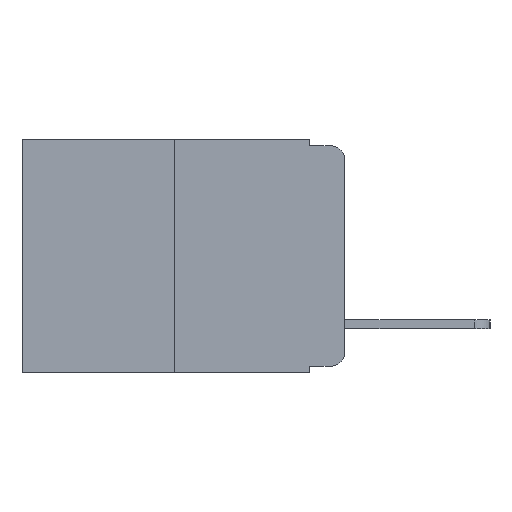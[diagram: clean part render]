
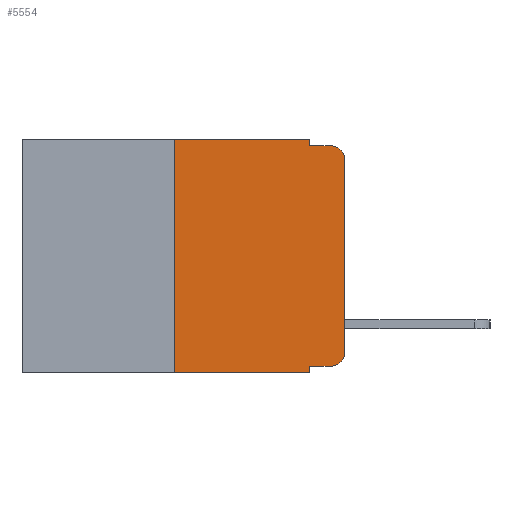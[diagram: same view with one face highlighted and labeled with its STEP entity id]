
A CAD part, left-side view. The second image highlights one B-rep face of the part: STEP entity #5554.
In plain terms, the highlighted planar face has unit normal (-1, 0, 0).
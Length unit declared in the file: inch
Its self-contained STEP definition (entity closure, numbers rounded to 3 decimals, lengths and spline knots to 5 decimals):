
#55 = EDGE_LOOP ( 'NONE', ( #23226, #8332, #12631, #1356, #17486, #22641, #6221, #17511, #11118, #7426 ) ) ;
#192 = VECTOR ( 'NONE', #3516, 39.37008 ) ;
#468 = CARTESIAN_POINT ( 'NONE',  ( 0., 0.02, -0.333 ) ) ;
#478 = VECTOR ( 'NONE', #23734, 39.37008 ) ;
#829 = EDGE_CURVE ( 'NONE', #23364, #8058, #15753, .T. ) ;
#837 = DIRECTION ( 'NONE',  ( -1., 0., 0. ) ) ;
#1308 = DIRECTION ( 'NONE',  ( -1., 0., 0. ) ) ;
#1338 = DIRECTION ( 'NONE',  ( 0., 0., -1. ) ) ;
#1356 = ORIENTED_EDGE ( 'NONE', *, *, #12495, .F. ) ;
#1454 = CARTESIAN_POINT ( 'NONE',  ( 0., 0.02, -0.03 ) ) ;
#2047 = CIRCLE ( 'NONE', #23955, 0.02 ) ;
#2201 = CARTESIAN_POINT ( 'NONE',  ( 0., 0.051, -0.333 ) ) ;
#3516 = DIRECTION ( 'NONE',  ( 0., 0., 1. ) ) ;
#3581 = CARTESIAN_POINT ( 'NONE',  ( 0., 0.473, 0. ) ) ;
#3917 = AXIS2_PLACEMENT_3D ( 'NONE', #19234, #21228, #9553 ) ;
#4253 = EDGE_CURVE ( 'NONE', #8058, #16435, #22614, .T. ) ;
#4354 = CARTESIAN_POINT ( 'NONE',  ( 0., 0.051, -0.343 ) ) ;
#4356 = LINE ( 'NONE', #15771, #24392 ) ;
#5285 = VECTOR ( 'NONE', #11398, 39.37008 ) ;
#5506 = DIRECTION ( 'NONE',  ( 0., -1., 0. ) ) ;
#5554 = ADVANCED_FACE ( 'NONE', ( #6406 ), #13431, .F. ) ;
#5944 = EDGE_CURVE ( 'NONE', #13067, #16435, #12203, .T. ) ;
#6221 = ORIENTED_EDGE ( 'NONE', *, *, #21981, .T. ) ;
#6253 = CARTESIAN_POINT ( 'NONE',  ( 0., 0., 0. ) ) ;
#6406 = FACE_OUTER_BOUND ( 'NONE', #55, .T. ) ;
#6565 = VERTEX_POINT ( 'NONE', #14674 ) ;
#6851 = LINE ( 'NONE', #21825, #478 ) ;
#7160 = CARTESIAN_POINT ( 'NONE',  ( 0., 0., -0.313 ) ) ;
#7342 = DIRECTION ( 'NONE',  ( 0., 0., -1. ) ) ;
#7426 = ORIENTED_EDGE ( 'NONE', *, *, #19051, .T. ) ;
#7667 = LINE ( 'NONE', #11842, #17429 ) ;
#8058 = VERTEX_POINT ( 'NONE', #21269 ) ;
#8332 = ORIENTED_EDGE ( 'NONE', *, *, #4253, .T. ) ;
#8640 = EDGE_CURVE ( 'NONE', #11841, #11509, #6851, .T. ) ;
#8820 = VECTOR ( 'NONE', #7342, 39.37008 ) ;
#9287 = LINE ( 'NONE', #25022, #24155 ) ;
#9553 = DIRECTION ( 'NONE',  ( 0., 0., -1. ) ) ;
#11118 = ORIENTED_EDGE ( 'NONE', *, *, #20085, .T. ) ;
#11398 = DIRECTION ( 'NONE',  ( 0., -1., 0. ) ) ;
#11509 = VERTEX_POINT ( 'NONE', #24253 ) ;
#11786 = CARTESIAN_POINT ( 'NONE',  ( 0., 0.25, -0.343 ) ) ;
#11840 = DIRECTION ( 'NONE',  ( 0., -1., 0. ) ) ;
#11841 = VERTEX_POINT ( 'NONE', #11786 ) ;
#11842 = CARTESIAN_POINT ( 'NONE',  ( 0., 0.051, 0. ) ) ;
#11906 = CARTESIAN_POINT ( 'NONE',  ( 0., 0.051, -0.01 ) ) ;
#12203 = LINE ( 'NONE', #24288, #17358 ) ;
#12495 = EDGE_CURVE ( 'NONE', #6565, #13067, #7667, .T. ) ;
#12499 = CARTESIAN_POINT ( 'NONE',  ( 0., 0.02, -0.313 ) ) ;
#12631 = ORIENTED_EDGE ( 'NONE', *, *, #5944, .F. ) ;
#13067 = VERTEX_POINT ( 'NONE', #11906 ) ;
#13287 = CARTESIAN_POINT ( 'NONE',  ( 0., 0.051, 0. ) ) ;
#13431 = PLANE ( 'NONE',  #3917 ) ;
#13839 = DIRECTION ( 'NONE',  ( 0., 0., -1. ) ) ;
#14497 = DIRECTION ( 'NONE',  ( 0., 0., -1. ) ) ;
#14672 = LINE ( 'NONE', #13287, #8820 ) ;
#14674 = CARTESIAN_POINT ( 'NONE',  ( 0., 0.051, 0. ) ) ;
#14913 = VERTEX_POINT ( 'NONE', #2201 ) ;
#15098 = LINE ( 'NONE', #3581, #5285 ) ;
#15753 = LINE ( 'NONE', #6253, #192 ) ;
#15771 = CARTESIAN_POINT ( 'NONE',  ( 0., 0.473, -0.343 ) ) ;
#16435 = VERTEX_POINT ( 'NONE', #20655 ) ;
#17358 = VECTOR ( 'NONE', #18468, 39.37008 ) ;
#17429 = VECTOR ( 'NONE', #13839, 39.37008 ) ;
#17476 = EDGE_CURVE ( 'NONE', #14913, #23680, #14672, .T. ) ;
#17486 = ORIENTED_EDGE ( 'NONE', *, *, #20573, .F. ) ;
#17511 = ORIENTED_EDGE ( 'NONE', *, *, #17476, .F. ) ;
#17702 = VERTEX_POINT ( 'NONE', #468 ) ;
#18468 = DIRECTION ( 'NONE',  ( 0., -1., 0. ) ) ;
#19051 = EDGE_CURVE ( 'NONE', #17702, #23364, #2047, .T. ) ;
#19234 = CARTESIAN_POINT ( 'NONE',  ( 0., 0.473, 0. ) ) ;
#20085 = EDGE_CURVE ( 'NONE', #14913, #17702, #9287, .T. ) ;
#20573 = EDGE_CURVE ( 'NONE', #11509, #6565, #15098, .T. ) ;
#20655 = CARTESIAN_POINT ( 'NONE',  ( 0., 0.02, -0.01 ) ) ;
#20695 = AXIS2_PLACEMENT_3D ( 'NONE', #1454, #1308, #1338 ) ;
#21228 = DIRECTION ( 'NONE',  ( 1., 0., 0. ) ) ;
#21269 = CARTESIAN_POINT ( 'NONE',  ( 0., 0., -0.03 ) ) ;
#21825 = CARTESIAN_POINT ( 'NONE',  ( 0., 0.25, 0. ) ) ;
#21981 = EDGE_CURVE ( 'NONE', #11841, #23680, #4356, .T. ) ;
#22614 = CIRCLE ( 'NONE', #20695, 0.02 ) ;
#22641 = ORIENTED_EDGE ( 'NONE', *, *, #8640, .F. ) ;
#23226 = ORIENTED_EDGE ( 'NONE', *, *, #829, .T. ) ;
#23364 = VERTEX_POINT ( 'NONE', #7160 ) ;
#23680 = VERTEX_POINT ( 'NONE', #4354 ) ;
#23734 = DIRECTION ( 'NONE',  ( 0., 0., 1. ) ) ;
#23955 = AXIS2_PLACEMENT_3D ( 'NONE', #12499, #837, #14497 ) ;
#24155 = VECTOR ( 'NONE', #5506, 39.37008 ) ;
#24253 = CARTESIAN_POINT ( 'NONE',  ( 0., 0.25, 0. ) ) ;
#24288 = CARTESIAN_POINT ( 'NONE',  ( 0., 0.051, -0.01 ) ) ;
#24392 = VECTOR ( 'NONE', #11840, 39.37008 ) ;
#25022 = CARTESIAN_POINT ( 'NONE',  ( 0., 0.051, -0.333 ) ) ;
